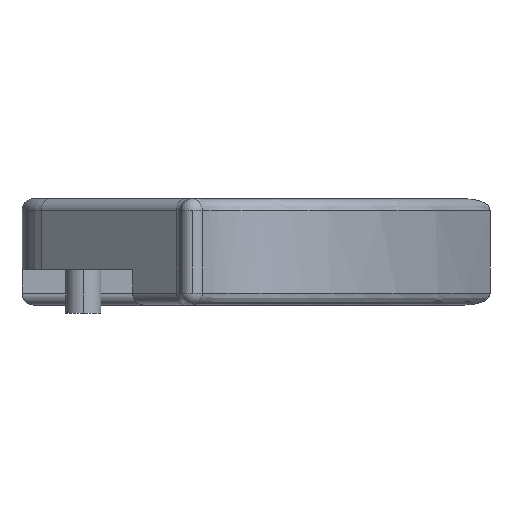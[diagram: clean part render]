
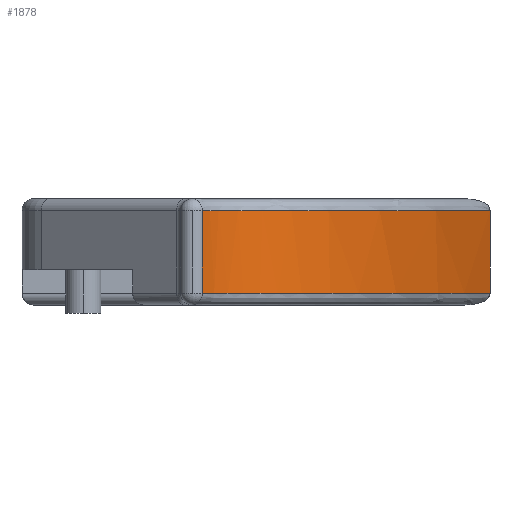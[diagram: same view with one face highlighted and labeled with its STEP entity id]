
A CAD part, left-side view. The second image highlights one B-rep face of the part: STEP entity #1878.
In plain terms, the highlighted free-form (B-spline) face has degree [3, 1] with [4, 2] control points.
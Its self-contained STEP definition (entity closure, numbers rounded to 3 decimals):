
#21 = EDGE_LOOP ( 'NONE', ( #1831, #1832, #1830, #1824 ) ) ;
#114 = B_SPLINE_CURVE_WITH_KNOTS ( 'NONE', 3,
 ( #1567, #1561, #1571, #1572, #1573, #1574, #1575, #1576, #1577, #1578, #1579, #1580, #1581, #1582, #1583, #1584, #1585, #1586, #1587, #1588, #1589, #1590, #1591, #1592, #1593, #1594, #1595, #1596 ),
 .UNSPECIFIED., .F., .F.,
 ( 4, 2, 2, 2, 2, 2, 2, 2, 2, 2, 2, 2, 2, 4 ),
 ( 0., 0.003, 0.007, 0.01, 0.012, 0.013, 0.015, 0.017, 0.02, 0.021, 0.022, 0.023, 0.025, 0.026 ),
 .UNSPECIFIED. ) ;
#115 = B_SPLINE_CURVE_WITH_KNOTS ( 'NONE', 3,
 ( #1569, #1570, #1598, #1599, #1600, #1601, #1602, #1603, #1604, #1605, #1606, #1607, #1608, #1609, #1610, #1611, #1612, #1613, #1614, #1615, #1616, #1617, #1618, #1619, #1620, #1621, #1622, #1623 ),
 .UNSPECIFIED., .F., .F.,
 ( 4, 2, 2, 2, 2, 2, 2, 2, 2, 2, 2, 2, 2, 4 ),
 ( 0., 0.002, 0.003, 0.005, 0.006, 0.007, 0.01, 0.012, 0.013, 0.015, 0.017, 0.02, 0.023, 0.027 ),
 .UNSPECIFIED. ) ;
#161 = FACE_OUTER_BOUND ( 'NONE', #21, .T. ) ;
#286 = LINE ( 'NONE', #1530, #288 ) ;
#288 = VECTOR ( 'NONE', #1526, 1000. ) ;
#308 = LINE ( 'NONE', #1566, #311 ) ;
#311 = VECTOR ( 'NONE', #1568, 1000. ) ;
#421 = CARTESIAN_POINT ( 'NONE',  ( 3.733, -1.816, 1. ) ) ;
#428 = CARTESIAN_POINT ( 'NONE',  ( 3.733, -1.816, 8. ) ) ;
#431 = CARTESIAN_POINT ( 'NONE',  ( 11., -6.971, 8. ) ) ;
#432 = CARTESIAN_POINT ( 'NONE',  ( 11., -6.971, 1. ) ) ;
#433 = CARTESIAN_POINT ( 'NONE',  ( 10.326, -18.653, 8. ) ) ;
#434 = CARTESIAN_POINT ( 'NONE',  ( 10.326, -18.653, 1. ) ) ;
#435 = CARTESIAN_POINT ( 'NONE',  ( 7.215, -26.178, 8. ) ) ;
#436 = CARTESIAN_POINT ( 'NONE',  ( 7.215, -26.178, 1. ) ) ;
#1193 = CARTESIAN_POINT ( 'NONE',  ( 3.733, -1.816, 1. ) ) ;
#1198 = CARTESIAN_POINT ( 'NONE',  ( 7.215, -26.178, 1. ) ) ;
#1248 = CARTESIAN_POINT ( 'NONE',  ( 7.215, -26.178, 8. ) ) ;
#1251 = CARTESIAN_POINT ( 'NONE',  ( 3.733, -1.816, 8. ) ) ;
#1526 = DIRECTION ( 'NONE',  ( 0., 0., -1. ) ) ;
#1530 = CARTESIAN_POINT ( 'NONE',  ( 3.733, -1.816, 8. ) ) ;
#1561 = CARTESIAN_POINT ( 'NONE',  ( 7.637, -25.159, 8. ) ) ;
#1566 = CARTESIAN_POINT ( 'NONE',  ( 7.215, -26.178, 9. ) ) ;
#1567 = CARTESIAN_POINT ( 'NONE',  ( 7.215, -26.178, 8. ) ) ;
#1568 = DIRECTION ( 'NONE',  ( 0., 0., -1. ) ) ;
#1569 = CARTESIAN_POINT ( 'NONE',  ( 3.733, -1.816, 1. ) ) ;
#1570 = CARTESIAN_POINT ( 'NONE',  ( 4.187, -2.138, 1. ) ) ;
#1571 = CARTESIAN_POINT ( 'NONE',  ( 7.994, -24.112, 8. ) ) ;
#1572 = CARTESIAN_POINT ( 'NONE',  ( 8.595, -21.986, 8. ) ) ;
#1573 = CARTESIAN_POINT ( 'NONE',  ( 8.836, -20.916, 8. ) ) ;
#1574 = CARTESIAN_POINT ( 'NONE',  ( 9.203, -18.76, 8. ) ) ;
#1575 = CARTESIAN_POINT ( 'NONE',  ( 9.33, -17.675, 8. ) ) ;
#1576 = CARTESIAN_POINT ( 'NONE',  ( 9.425, -16.036, 8. ) ) ;
#1577 = CARTESIAN_POINT ( 'NONE',  ( 9.44, -15.487, 8. ) ) ;
#1578 = CARTESIAN_POINT ( 'NONE',  ( 9.437, -14.385, 8. ) ) ;
#1579 = CARTESIAN_POINT ( 'NONE',  ( 9.417, -13.831, 8. ) ) ;
#1580 = CARTESIAN_POINT ( 'NONE',  ( 9.339, -12.729, 8. ) ) ;
#1581 = CARTESIAN_POINT ( 'NONE',  ( 9.281, -12.179, 8. ) ) ;
#1582 = CARTESIAN_POINT ( 'NONE',  ( 9.122, -11.085, 8. ) ) ;
#1583 = CARTESIAN_POINT ( 'NONE',  ( 9.02, -10.54, 8. ) ) ;
#1584 = CARTESIAN_POINT ( 'NONE',  ( 8.647, -8.932, 8. ) ) ;
#1585 = CARTESIAN_POINT ( 'NONE',  ( 8.306, -7.89, 8. ) ) ;
#1586 = CARTESIAN_POINT ( 'NONE',  ( 7.733, -6.633, 8. ) ) ;
#1587 = CARTESIAN_POINT ( 'NONE',  ( 7.61, -6.383, 8. ) ) ;
#1588 = CARTESIAN_POINT ( 'NONE',  ( 7.352, -5.894, 8. ) ) ;
#1589 = CARTESIAN_POINT ( 'NONE',  ( 7.216, -5.655, 8. ) ) ;
#1590 = CARTESIAN_POINT ( 'NONE',  ( 6.788, -4.953, 8. ) ) ;
#1591 = CARTESIAN_POINT ( 'NONE',  ( 6.476, -4.506, 8. ) ) ;
#1592 = CARTESIAN_POINT ( 'NONE',  ( 5.793, -3.655, 8. ) ) ;
#1593 = CARTESIAN_POINT ( 'NONE',  ( 5.422, -3.252, 8. ) ) ;
#1594 = CARTESIAN_POINT ( 'NONE',  ( 4.619, -2.492, 8. ) ) ;
#1595 = CARTESIAN_POINT ( 'NONE',  ( 4.187, -2.138, 8. ) ) ;
#1596 = CARTESIAN_POINT ( 'NONE',  ( 3.733, -1.816, 8. ) ) ;
#1598 = CARTESIAN_POINT ( 'NONE',  ( 4.619, -2.492, 1. ) ) ;
#1599 = CARTESIAN_POINT ( 'NONE',  ( 5.422, -3.252, 1. ) ) ;
#1600 = CARTESIAN_POINT ( 'NONE',  ( 5.793, -3.655, 1. ) ) ;
#1601 = CARTESIAN_POINT ( 'NONE',  ( 6.476, -4.506, 1. ) ) ;
#1602 = CARTESIAN_POINT ( 'NONE',  ( 6.788, -4.953, 1. ) ) ;
#1603 = CARTESIAN_POINT ( 'NONE',  ( 7.216, -5.655, 1. ) ) ;
#1604 = CARTESIAN_POINT ( 'NONE',  ( 7.352, -5.894, 1. ) ) ;
#1605 = CARTESIAN_POINT ( 'NONE',  ( 7.61, -6.383, 1. ) ) ;
#1606 = CARTESIAN_POINT ( 'NONE',  ( 7.733, -6.633, 1. ) ) ;
#1607 = CARTESIAN_POINT ( 'NONE',  ( 8.306, -7.89, 1. ) ) ;
#1608 = CARTESIAN_POINT ( 'NONE',  ( 8.647, -8.932, 1. ) ) ;
#1609 = CARTESIAN_POINT ( 'NONE',  ( 9.02, -10.54, 1. ) ) ;
#1610 = CARTESIAN_POINT ( 'NONE',  ( 9.122, -11.085, 1. ) ) ;
#1611 = CARTESIAN_POINT ( 'NONE',  ( 9.281, -12.179, 1. ) ) ;
#1612 = CARTESIAN_POINT ( 'NONE',  ( 9.339, -12.729, 1. ) ) ;
#1613 = CARTESIAN_POINT ( 'NONE',  ( 9.417, -13.831, 1. ) ) ;
#1614 = CARTESIAN_POINT ( 'NONE',  ( 9.437, -14.385, 1. ) ) ;
#1615 = CARTESIAN_POINT ( 'NONE',  ( 9.44, -15.487, 1. ) ) ;
#1616 = CARTESIAN_POINT ( 'NONE',  ( 9.425, -16.036, 1. ) ) ;
#1617 = CARTESIAN_POINT ( 'NONE',  ( 9.33, -17.675, 1. ) ) ;
#1618 = CARTESIAN_POINT ( 'NONE',  ( 9.203, -18.76, 1. ) ) ;
#1619 = CARTESIAN_POINT ( 'NONE',  ( 8.836, -20.916, 1. ) ) ;
#1620 = CARTESIAN_POINT ( 'NONE',  ( 8.595, -21.986, 1. ) ) ;
#1621 = CARTESIAN_POINT ( 'NONE',  ( 7.994, -24.112, 1. ) ) ;
#1622 = CARTESIAN_POINT ( 'NONE',  ( 7.637, -25.157, 1. ) ) ;
#1623 = CARTESIAN_POINT ( 'NONE',  ( 7.215, -26.178, 1. ) ) ;
#1824 = ORIENTED_EDGE ( 'NONE', *, *, #2340, .T. ) ;
#1830 = ORIENTED_EDGE ( 'NONE', *, *, #2324, .T. ) ;
#1831 = ORIENTED_EDGE ( 'NONE', *, *, #2338, .F. ) ;
#1832 = ORIENTED_EDGE ( 'NONE', *, *, #2339, .T. ) ;
#1878 = ADVANCED_FACE ( 'NONE', ( #161 ), #2382, .F. ) ;
#1913 = VERTEX_POINT ( 'NONE', #1193 ) ;
#1918 = VERTEX_POINT ( 'NONE', #1198 ) ;
#2204 = VERTEX_POINT ( 'NONE', #1248 ) ;
#2209 = VERTEX_POINT ( 'NONE', #1251 ) ;
#2324 = EDGE_CURVE ( 'NONE', #2209, #1913, #286, .T. ) ;
#2338 = EDGE_CURVE ( 'NONE', #2204, #1918, #308, .T. ) ;
#2339 = EDGE_CURVE ( 'NONE', #2204, #2209, #114, .T. ) ;
#2340 = EDGE_CURVE ( 'NONE', #1913, #1918, #115, .T. ) ;
#2382 = B_SPLINE_SURFACE_WITH_KNOTS ( 'NONE', 3, 1, ( 
 ( #428, #421 ),
 ( #431, #432 ),
 ( #433, #434 ),
 ( #435, #436 ) ),
 .UNSPECIFIED., .F., .F., .F.,
 ( 4, 4 ),
 ( 2, 2 ),
 ( 0.128, 1. ),
 ( 0., 1. ),
 .UNSPECIFIED. ) ;
